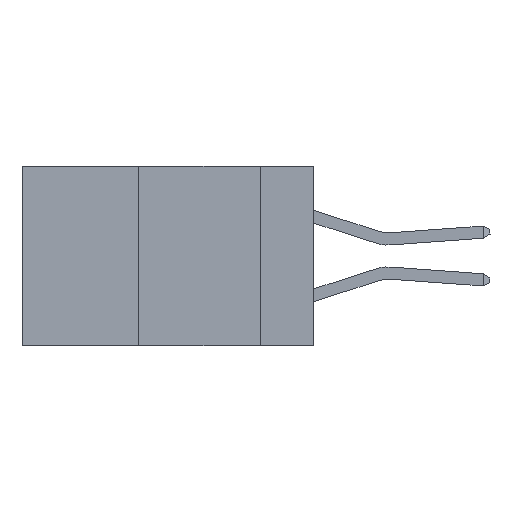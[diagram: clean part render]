
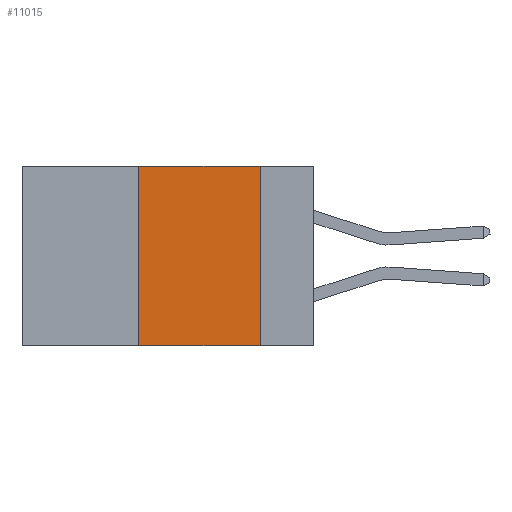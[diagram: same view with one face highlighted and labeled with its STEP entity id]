
A CAD part, left-side view. The second image highlights one B-rep face of the part: STEP entity #11015.
In plain terms, the highlighted planar face has unit normal (-1, 0, 0).
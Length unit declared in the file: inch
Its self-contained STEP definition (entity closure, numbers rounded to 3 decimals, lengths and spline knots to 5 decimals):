
#1010 = CARTESIAN_POINT ( 'NONE',  ( 0., 0.36, 0. ) ) ;
#1066 = EDGE_CURVE ( 'NONE', #10548, #19180, #15158, .T. ) ;
#1155 = VECTOR ( 'NONE', #22583, 39.37008 ) ;
#1163 = DIRECTION ( 'NONE',  ( 0., 0., -1. ) ) ;
#1694 = LINE ( 'NONE', #24477, #1155 ) ;
#2172 = CARTESIAN_POINT ( 'NONE',  ( 0., 0.11, -0.37 ) ) ;
#2811 = CARTESIAN_POINT ( 'NONE',  ( 0., 0.36, -0.37 ) ) ;
#2937 = DIRECTION ( 'NONE',  ( 0., 0., -1. ) ) ;
#3324 = EDGE_CURVE ( 'NONE', #19180, #14829, #21508, .T. ) ;
#4799 = DIRECTION ( 'NONE',  ( 1., 0., 0. ) ) ;
#5149 = LINE ( 'NONE', #1010, #6821 ) ;
#6821 = VECTOR ( 'NONE', #15088, 39.37008 ) ;
#7243 = DIRECTION ( 'NONE',  ( 0., -1., 0. ) ) ;
#7438 = FACE_OUTER_BOUND ( 'NONE', #10822, .T. ) ;
#8583 = CARTESIAN_POINT ( 'NONE',  ( 0., 0.36, 0. ) ) ;
#10548 = VERTEX_POINT ( 'NONE', #8583 ) ;
#10822 = EDGE_LOOP ( 'NONE', ( #15229, #21806, #12081, #19535 ) ) ;
#11015 = ADVANCED_FACE ( 'NONE', ( #7438 ), #21290, .F. ) ;
#12081 = ORIENTED_EDGE ( 'NONE', *, *, #24381, .F. ) ;
#14731 = VERTEX_POINT ( 'NONE', #2811 ) ;
#14829 = VERTEX_POINT ( 'NONE', #2172 ) ;
#15088 = DIRECTION ( 'NONE',  ( 0., 0., 1. ) ) ;
#15158 = LINE ( 'NONE', #25613, #17316 ) ;
#15229 = ORIENTED_EDGE ( 'NONE', *, *, #3324, .F. ) ;
#17316 = VECTOR ( 'NONE', #7243, 39.37008 ) ;
#18883 = CARTESIAN_POINT ( 'NONE',  ( 0., 0.6, 0. ) ) ;
#19180 = VERTEX_POINT ( 'NONE', #24265 ) ;
#19370 = CARTESIAN_POINT ( 'NONE',  ( 0., 0.11, 0. ) ) ;
#19535 = ORIENTED_EDGE ( 'NONE', *, *, #20084, .T. ) ;
#20084 = EDGE_CURVE ( 'NONE', #14731, #14829, #1694, .T. ) ;
#21290 = PLANE ( 'NONE',  #26244 ) ;
#21508 = LINE ( 'NONE', #19370, #25928 ) ;
#21806 = ORIENTED_EDGE ( 'NONE', *, *, #1066, .F. ) ;
#22583 = DIRECTION ( 'NONE',  ( 0., -1., 0. ) ) ;
#24265 = CARTESIAN_POINT ( 'NONE',  ( 0., 0.11, 0. ) ) ;
#24381 = EDGE_CURVE ( 'NONE', #14731, #10548, #5149, .T. ) ;
#24477 = CARTESIAN_POINT ( 'NONE',  ( 0., 0.6, -0.37 ) ) ;
#25613 = CARTESIAN_POINT ( 'NONE',  ( 0., 0.6, 0. ) ) ;
#25928 = VECTOR ( 'NONE', #1163, 39.37008 ) ;
#26244 = AXIS2_PLACEMENT_3D ( 'NONE', #18883, #4799, #2937 ) ;
